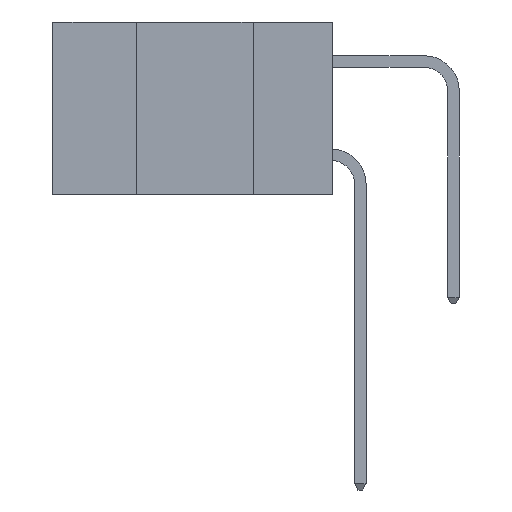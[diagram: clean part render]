
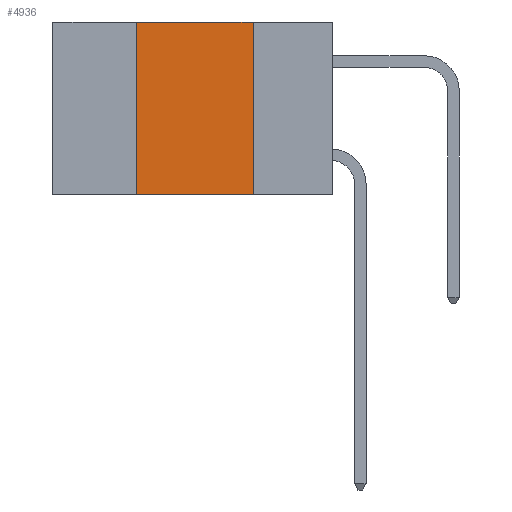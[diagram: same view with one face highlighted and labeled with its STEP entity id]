
A CAD part, left-side view. The second image highlights one B-rep face of the part: STEP entity #4936.
In plain terms, the highlighted planar face has unit normal (-1, 0, 0).
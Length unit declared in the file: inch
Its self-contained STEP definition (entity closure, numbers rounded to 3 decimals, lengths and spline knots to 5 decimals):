
#111 = CARTESIAN_POINT ( 'NONE',  ( 0., 0.42, 0. ) ) ;
#197 = CARTESIAN_POINT ( 'NONE',  ( 0., 0.17, -0.37 ) ) ;
#316 = CARTESIAN_POINT ( 'NONE',  ( 0., 0.17, -0.37 ) ) ;
#1014 = LINE ( 'NONE', #7926, #3704 ) ;
#1714 = VECTOR ( 'NONE', #6741, 39.37008 ) ;
#1761 = EDGE_LOOP ( 'NONE', ( #9019, #3326, #2997, #4825 ) ) ;
#2111 = AXIS2_PLACEMENT_3D ( 'NONE', #2642, #7794, #2775 ) ;
#2434 = DIRECTION ( 'NONE',  ( 0., -1., 0. ) ) ;
#2535 = LINE ( 'NONE', #3541, #10315 ) ;
#2642 = CARTESIAN_POINT ( 'NONE',  ( 0., 0.6, 0. ) ) ;
#2775 = DIRECTION ( 'NONE',  ( 0., 0., -1. ) ) ;
#2997 = ORIENTED_EDGE ( 'NONE', *, *, #4019, .F. ) ;
#3326 = ORIENTED_EDGE ( 'NONE', *, *, #9749, .F. ) ;
#3541 = CARTESIAN_POINT ( 'NONE',  ( 0., 0.6, -0.37 ) ) ;
#3704 = VECTOR ( 'NONE', #11107, 39.37008 ) ;
#4019 = EDGE_CURVE ( 'NONE', #7135, #6969, #4439, .T. ) ;
#4057 = CARTESIAN_POINT ( 'NONE',  ( 0., 0.42, -0.37 ) ) ;
#4439 = LINE ( 'NONE', #7415, #1714 ) ;
#4825 = ORIENTED_EDGE ( 'NONE', *, *, #12214, .T. ) ;
#4936 = ADVANCED_FACE ( 'NONE', ( #5525 ), #8832, .F. ) ;
#5525 = FACE_OUTER_BOUND ( 'NONE', #1761, .T. ) ;
#6286 = LINE ( 'NONE', #197, #11379 ) ;
#6741 = DIRECTION ( 'NONE',  ( 0., 0., 1. ) ) ;
#6969 = VERTEX_POINT ( 'NONE', #111 ) ;
#7034 = EDGE_CURVE ( 'NONE', #8958, #8271, #6286, .T. ) ;
#7135 = VERTEX_POINT ( 'NONE', #4057 ) ;
#7415 = CARTESIAN_POINT ( 'NONE',  ( 0., 0.42, -0.37 ) ) ;
#7794 = DIRECTION ( 'NONE',  ( 1., 0., 0. ) ) ;
#7926 = CARTESIAN_POINT ( 'NONE',  ( 0., 0.6, 0. ) ) ;
#8271 = VERTEX_POINT ( 'NONE', #316 ) ;
#8832 = PLANE ( 'NONE',  #2111 ) ;
#8958 = VERTEX_POINT ( 'NONE', #10466 ) ;
#9019 = ORIENTED_EDGE ( 'NONE', *, *, #7034, .F. ) ;
#9749 = EDGE_CURVE ( 'NONE', #6969, #8958, #1014, .T. ) ;
#10315 = VECTOR ( 'NONE', #2434, 39.37008 ) ;
#10466 = CARTESIAN_POINT ( 'NONE',  ( 0., 0.17, 0. ) ) ;
#11107 = DIRECTION ( 'NONE',  ( 0., -1., 0. ) ) ;
#11379 = VECTOR ( 'NONE', #11492, 39.37008 ) ;
#11492 = DIRECTION ( 'NONE',  ( 0., 0., -1. ) ) ;
#12214 = EDGE_CURVE ( 'NONE', #7135, #8271, #2535, .T. ) ;
